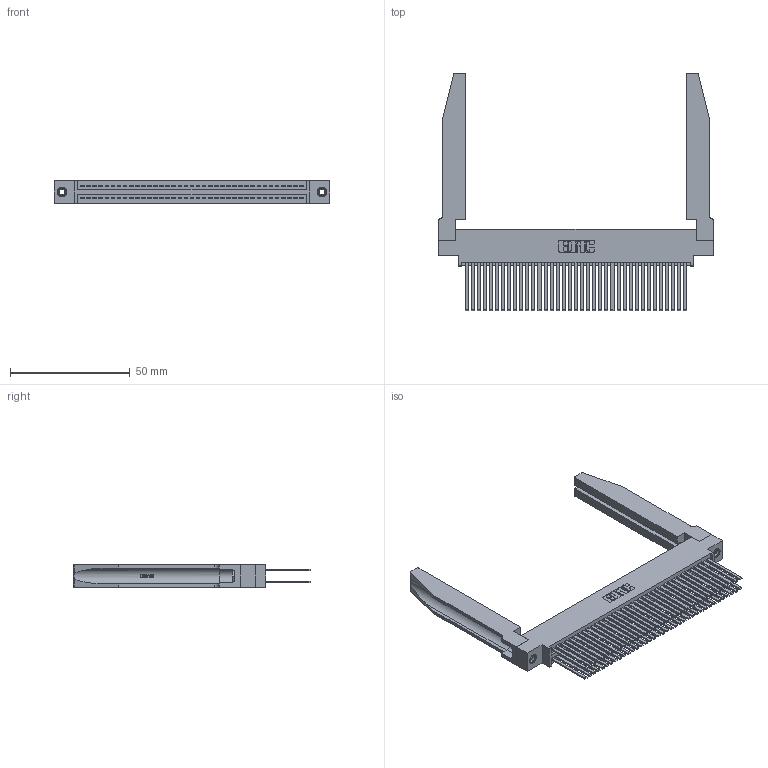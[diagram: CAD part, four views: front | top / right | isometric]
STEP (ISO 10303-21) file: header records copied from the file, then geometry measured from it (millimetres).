
FILE_DESCRIPTION (( 'STEP AP203' ), '1' );
FILE_NAME ('395-074-544-878.STEP', '2019-10-24T14:51:57', ( '' ), ( '' ), 'SwSTEP 2.0', 'SolidWorks 2016', '' );
FILE_SCHEMA (( 'CONFIG_CONTROL_DESIGN' ));
Length unit declared in the file: inch
Products named in the file (5): 345-292-001_345-293-144; 345-250-001_345-250-001-102; 345-220-078_345-220-078; 395-074-544-878; 345 Part_0.170 Offset - 0.156 Dia-TH
Assembly tree (79 placements, depth 2):
  395-074-544-878
    345 Part_0.170 Offset - 0.156 Dia-TH
    345-292-001_345-293-144  x74
    345-250-001_345-250-001-102  x2
    345-220-078_345-220-078  x2
Bounding box: 115.21 x 99.24 x 9.4 mm (x, y, z)
Volume: 19840 mm3; surface area: 27766.3 mm2
Topology: 79 solids, 79 shells, 3620 faces, 10655 edges, 6994 vertices
Faces by surface type: plane 2372, cylinder 1196, bspline 36, cone 12, torus 4
Entity records: 34392 total; most frequent: CARTESIAN_POINT 6687, ORIENTED_EDGE 5518, DIRECTION 4893, EDGE_CURVE 2759, VECTOR 2389, LINE 2389, VERTEX_POINT 1832, AXIS2_PLACEMENT_3D 1252
